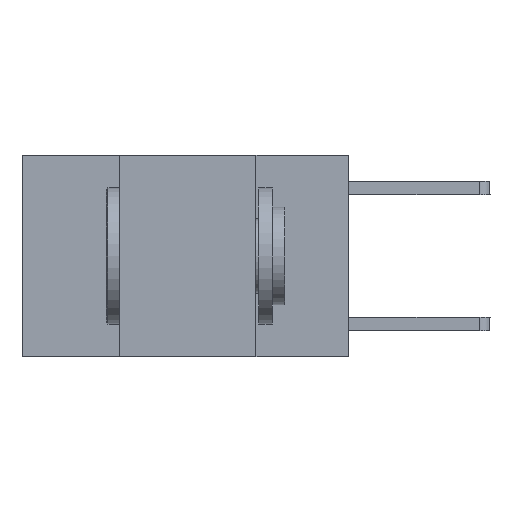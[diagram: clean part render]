
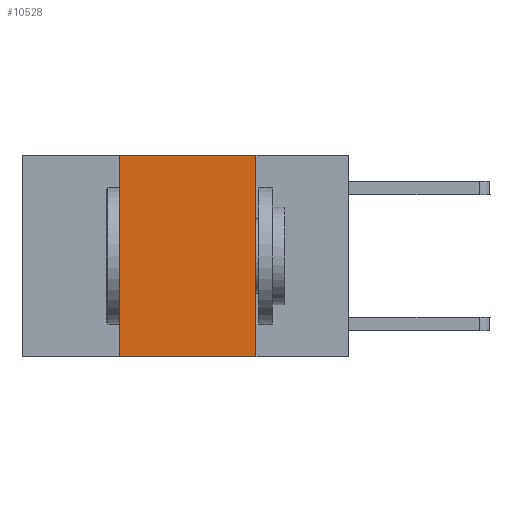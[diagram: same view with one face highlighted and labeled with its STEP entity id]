
A CAD part, left-side view. The second image highlights one B-rep face of the part: STEP entity #10528.
In plain terms, the highlighted planar face has unit normal (-1, 0, 0).
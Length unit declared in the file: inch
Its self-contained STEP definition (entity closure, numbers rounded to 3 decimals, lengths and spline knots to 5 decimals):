
#59 = EDGE_CURVE ( 'NONE', #4473, #6842, #949, .T. ) ;
#893 = CARTESIAN_POINT ( 'NONE',  ( 0., 0.17, 0. ) ) ;
#949 = LINE ( 'NONE', #893, #1228 ) ;
#1174 = EDGE_LOOP ( 'NONE', ( #2284, #6399, #6967, #7047 ) ) ;
#1228 = VECTOR ( 'NONE', #6062, 39.37008 ) ;
#1332 = VERTEX_POINT ( 'NONE', #6652 ) ;
#1494 = EDGE_CURVE ( 'NONE', #5075, #1332, #2621, .T. ) ;
#1627 = DIRECTION ( 'NONE',  ( 0., -1., 0. ) ) ;
#1669 = CARTESIAN_POINT ( 'NONE',  ( 0., 0.6, 0. ) ) ;
#1677 = CARTESIAN_POINT ( 'NONE',  ( 0., 0.42, 0. ) ) ;
#1723 = CARTESIAN_POINT ( 'NONE',  ( 0., 0.17, -0.37 ) ) ;
#2284 = ORIENTED_EDGE ( 'NONE', *, *, #59, .F. ) ;
#2529 = DIRECTION ( 'NONE',  ( 0., -1., 0. ) ) ;
#2621 = LINE ( 'NONE', #1677, #7293 ) ;
#4473 = VERTEX_POINT ( 'NONE', #6291 ) ;
#5075 = VERTEX_POINT ( 'NONE', #11036 ) ;
#5135 = VECTOR ( 'NONE', #1627, 39.37008 ) ;
#5807 = EDGE_CURVE ( 'NONE', #1332, #4473, #6921, .T. ) ;
#6062 = DIRECTION ( 'NONE',  ( 0., 0., -1. ) ) ;
#6063 = PLANE ( 'NONE',  #6513 ) ;
#6291 = CARTESIAN_POINT ( 'NONE',  ( 0., 0.17, 0. ) ) ;
#6399 = ORIENTED_EDGE ( 'NONE', *, *, #5807, .F. ) ;
#6513 = AXIS2_PLACEMENT_3D ( 'NONE', #1669, #6765, #6826 ) ;
#6652 = CARTESIAN_POINT ( 'NONE',  ( 0., 0.42, 0. ) ) ;
#6765 = DIRECTION ( 'NONE',  ( 1., 0., 0. ) ) ;
#6826 = DIRECTION ( 'NONE',  ( 0., 0., -1. ) ) ;
#6842 = VERTEX_POINT ( 'NONE', #1723 ) ;
#6921 = LINE ( 'NONE', #8839, #8140 ) ;
#6967 = ORIENTED_EDGE ( 'NONE', *, *, #1494, .F. ) ;
#7047 = ORIENTED_EDGE ( 'NONE', *, *, #8123, .T. ) ;
#7293 = VECTOR ( 'NONE', #10696, 39.37008 ) ;
#7605 = CARTESIAN_POINT ( 'NONE',  ( 0., 0.6, -0.37 ) ) ;
#8123 = EDGE_CURVE ( 'NONE', #5075, #6842, #8698, .T. ) ;
#8140 = VECTOR ( 'NONE', #2529, 39.37008 ) ;
#8698 = LINE ( 'NONE', #7605, #5135 ) ;
#8839 = CARTESIAN_POINT ( 'NONE',  ( 0., 0.6, 0. ) ) ;
#9611 = FACE_OUTER_BOUND ( 'NONE', #1174, .T. ) ;
#10528 = ADVANCED_FACE ( 'NONE', ( #9611 ), #6063, .F. ) ;
#10696 = DIRECTION ( 'NONE',  ( 0., 0., 1. ) ) ;
#11036 = CARTESIAN_POINT ( 'NONE',  ( 0., 0.42, -0.37 ) ) ;
